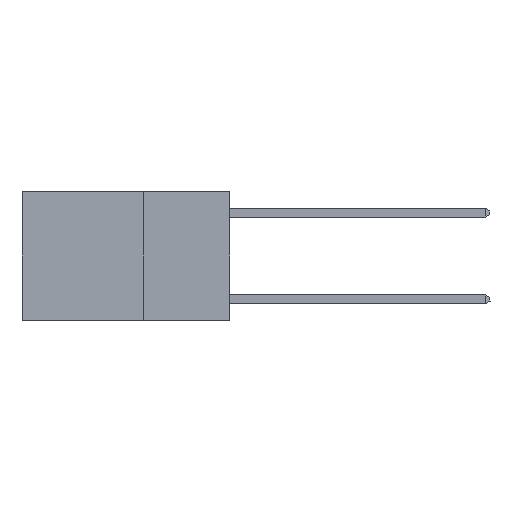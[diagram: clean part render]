
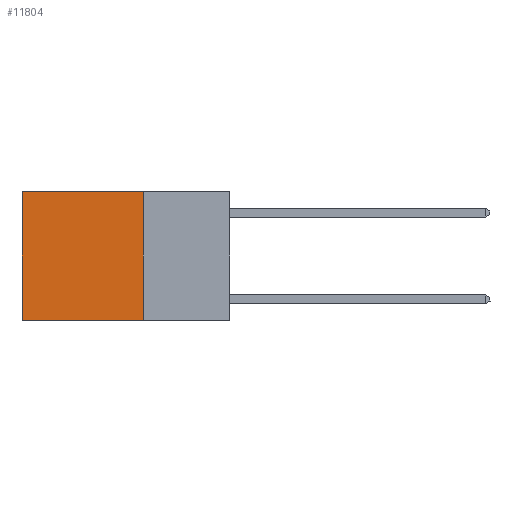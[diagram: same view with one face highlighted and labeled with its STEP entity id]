
A CAD part, left-side view. The second image highlights one B-rep face of the part: STEP entity #11804.
In plain terms, the highlighted planar face has unit normal (-1, 0, 0).
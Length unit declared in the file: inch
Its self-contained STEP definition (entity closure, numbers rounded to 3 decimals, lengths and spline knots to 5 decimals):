
#12 = CARTESIAN_POINT ( 'NONE',  ( 0.2625, 0.25, -0.37 ) ) ;
#1136 = CARTESIAN_POINT ( 'NONE',  ( 0.2625, 0.6, 0. ) ) ;
#1369 = CARTESIAN_POINT ( 'NONE',  ( 0.2625, 0.6, -0.37 ) ) ;
#2211 = VERTEX_POINT ( 'NONE', #3873 ) ;
#2621 = VERTEX_POINT ( 'NONE', #1369 ) ;
#3691 = ORIENTED_EDGE ( 'NONE', *, *, #7126, .F. ) ;
#3806 = EDGE_CURVE ( 'NONE', #10460, #2621, #20623, .T. ) ;
#3847 = LINE ( 'NONE', #13529, #6891 ) ;
#3873 = CARTESIAN_POINT ( 'NONE',  ( 0.2625, 0.25, 0. ) ) ;
#4260 = EDGE_CURVE ( 'NONE', #16896, #2621, #10789, .T. ) ;
#5092 = DIRECTION ( 'NONE',  ( 0., 0., -1. ) ) ;
#5420 = AXIS2_PLACEMENT_3D ( 'NONE', #7950, #10987, #11195 ) ;
#6891 = VECTOR ( 'NONE', #16873, 39.37008 ) ;
#7126 = EDGE_CURVE ( 'NONE', #2211, #16896, #14255, .T. ) ;
#7950 = CARTESIAN_POINT ( 'NONE',  ( 0.2625, 0.25, 0. ) ) ;
#9469 = EDGE_CURVE ( 'NONE', #2211, #10460, #3847, .T. ) ;
#9986 = VECTOR ( 'NONE', #11909, 39.37008 ) ;
#10042 = ORIENTED_EDGE ( 'NONE', *, *, #4260, .F. ) ;
#10460 = VERTEX_POINT ( 'NONE', #1136 ) ;
#10789 = LINE ( 'NONE', #12, #15550 ) ;
#10987 = DIRECTION ( 'NONE',  ( 1., 0., 0. ) ) ;
#11195 = DIRECTION ( 'NONE',  ( 0., 0., -1. ) ) ;
#11464 = ORIENTED_EDGE ( 'NONE', *, *, #3806, .T. ) ;
#11804 = ADVANCED_FACE ( 'NONE', ( #16836 ), #18549, .F. ) ;
#11909 = DIRECTION ( 'NONE',  ( 0., 0., -1. ) ) ;
#12044 = EDGE_LOOP ( 'NONE', ( #11464, #10042, #3691, #20610 ) ) ;
#12838 = DIRECTION ( 'NONE',  ( 0., 1., 0. ) ) ;
#13207 = CARTESIAN_POINT ( 'NONE',  ( 0.2625, 0.6, 0. ) ) ;
#13529 = CARTESIAN_POINT ( 'NONE',  ( 0.2625, 0.25, 0. ) ) ;
#14255 = LINE ( 'NONE', #19985, #9986 ) ;
#15550 = VECTOR ( 'NONE', #12838, 39.37008 ) ;
#16836 = FACE_OUTER_BOUND ( 'NONE', #12044, .T. ) ;
#16873 = DIRECTION ( 'NONE',  ( 0., 1., 0. ) ) ;
#16896 = VERTEX_POINT ( 'NONE', #20453 ) ;
#17836 = VECTOR ( 'NONE', #5092, 39.37008 ) ;
#18549 = PLANE ( 'NONE',  #5420 ) ;
#19985 = CARTESIAN_POINT ( 'NONE',  ( 0.2625, 0.25, 0. ) ) ;
#20453 = CARTESIAN_POINT ( 'NONE',  ( 0.2625, 0.25, -0.37 ) ) ;
#20610 = ORIENTED_EDGE ( 'NONE', *, *, #9469, .T. ) ;
#20623 = LINE ( 'NONE', #13207, #17836 ) ;
